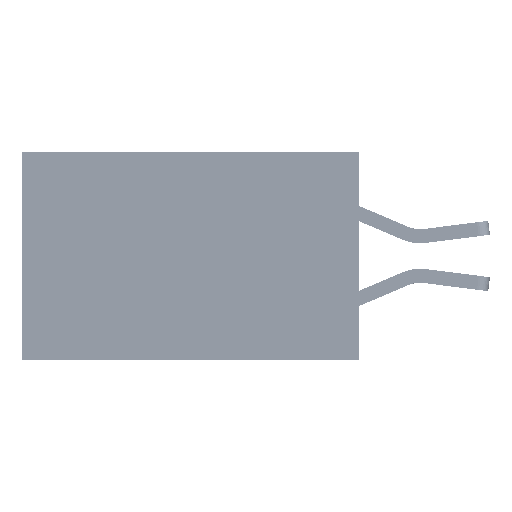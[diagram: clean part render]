
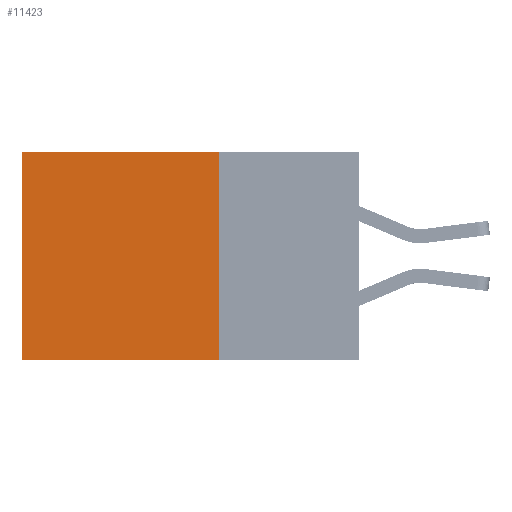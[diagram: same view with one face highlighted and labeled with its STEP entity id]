
A CAD part, left-side view. The second image highlights one B-rep face of the part: STEP entity #11423.
In plain terms, the highlighted planar face has unit normal (-1, 0, 0).
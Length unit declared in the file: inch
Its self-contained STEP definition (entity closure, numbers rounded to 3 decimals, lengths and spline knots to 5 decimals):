
#1476 = AXIS2_PLACEMENT_3D ( 'NONE', #5328, #5860, #30519 ) ;
#2210 = DIRECTION ( 'NONE',  ( 0., 0., -1. ) ) ;
#2950 = VERTEX_POINT ( 'NONE', #5479 ) ;
#5110 = VECTOR ( 'NONE', #2210, 39.37008 ) ;
#5328 = CARTESIAN_POINT ( 'NONE',  ( 0.2875, 0.25, 0. ) ) ;
#5479 = CARTESIAN_POINT ( 'NONE',  ( 0.2875, 0.25, 0. ) ) ;
#5757 = CARTESIAN_POINT ( 'NONE',  ( 0.2875, 0.25, -0.37 ) ) ;
#5860 = DIRECTION ( 'NONE',  ( 1., 0., 0. ) ) ;
#8100 = VERTEX_POINT ( 'NONE', #5757 ) ;
#9973 = PLANE ( 'NONE',  #1476 ) ;
#11417 = LINE ( 'NONE', #16174, #26868 ) ;
#11423 = ADVANCED_FACE ( 'NONE', ( #51542 ), #9973, .F. ) ;
#13586 = CARTESIAN_POINT ( 'NONE',  ( 0.2875, 0.25, -0.37 ) ) ;
#14473 = VERTEX_POINT ( 'NONE', #32325 ) ;
#14987 = ORIENTED_EDGE ( 'NONE', *, *, #45094, .F. ) ;
#16174 = CARTESIAN_POINT ( 'NONE',  ( 0.2875, 0.25, 0. ) ) ;
#19008 = EDGE_CURVE ( 'NONE', #14473, #40605, #28315, .T. ) ;
#20935 = LINE ( 'NONE', #13586, #24195 ) ;
#23848 = ORIENTED_EDGE ( 'NONE', *, *, #44254, .T. ) ;
#24195 = VECTOR ( 'NONE', #26387, 39.37008 ) ;
#25576 = LINE ( 'NONE', #27076, #44818 ) ;
#26208 = ORIENTED_EDGE ( 'NONE', *, *, #19008, .T. ) ;
#26321 = CARTESIAN_POINT ( 'NONE',  ( 0.2875, 0.6, 0. ) ) ;
#26387 = DIRECTION ( 'NONE',  ( 0., 1., 0. ) ) ;
#26868 = VECTOR ( 'NONE', #33089, 39.37008 ) ;
#27076 = CARTESIAN_POINT ( 'NONE',  ( 0.2875, 0.25, 0. ) ) ;
#28315 = LINE ( 'NONE', #26321, #5110 ) ;
#30519 = DIRECTION ( 'NONE',  ( 0., 0., -1. ) ) ;
#31182 = ORIENTED_EDGE ( 'NONE', *, *, #35975, .F. ) ;
#32325 = CARTESIAN_POINT ( 'NONE',  ( 0.2875, 0.6, 0. ) ) ;
#33089 = DIRECTION ( 'NONE',  ( 0., 1., 0. ) ) ;
#35975 = EDGE_CURVE ( 'NONE', #2950, #8100, #25576, .T. ) ;
#40605 = VERTEX_POINT ( 'NONE', #49957 ) ;
#44254 = EDGE_CURVE ( 'NONE', #2950, #14473, #11417, .T. ) ;
#44818 = VECTOR ( 'NONE', #47788, 39.37008 ) ;
#45094 = EDGE_CURVE ( 'NONE', #8100, #40605, #20935, .T. ) ;
#47788 = DIRECTION ( 'NONE',  ( 0., 0., -1. ) ) ;
#49957 = CARTESIAN_POINT ( 'NONE',  ( 0.2875, 0.6, -0.37 ) ) ;
#51379 = EDGE_LOOP ( 'NONE', ( #26208, #14987, #31182, #23848 ) ) ;
#51542 = FACE_OUTER_BOUND ( 'NONE', #51379, .T. ) ;
